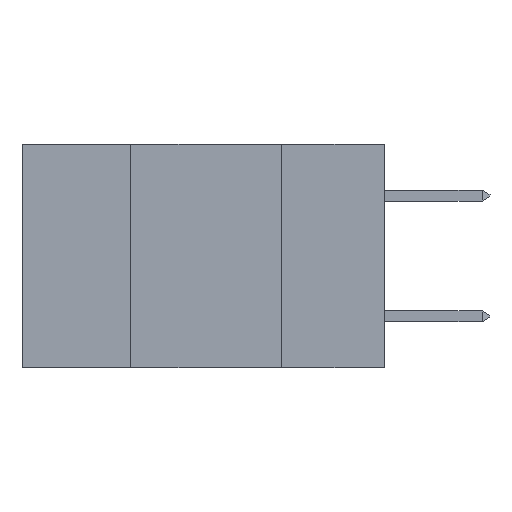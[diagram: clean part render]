
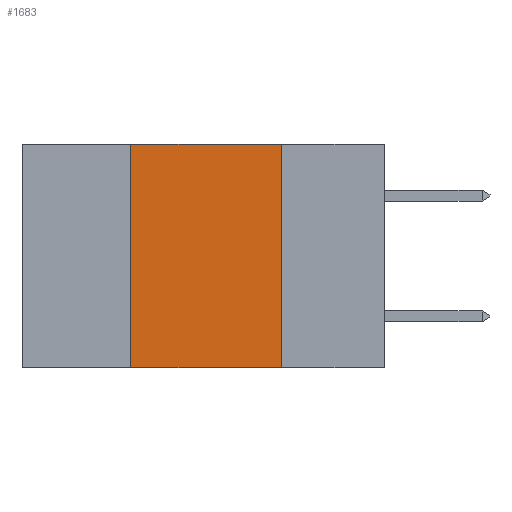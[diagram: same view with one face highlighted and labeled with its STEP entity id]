
A CAD part, left-side view. The second image highlights one B-rep face of the part: STEP entity #1683.
In plain terms, the highlighted planar face has unit normal (-1, 0, 0).
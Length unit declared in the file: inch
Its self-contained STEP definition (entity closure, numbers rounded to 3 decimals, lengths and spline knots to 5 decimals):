
#314 = CARTESIAN_POINT ( 'NONE',  ( 0., 0.42, 0. ) ) ;
#368 = VERTEX_POINT ( 'NONE', #5541 ) ;
#703 = CARTESIAN_POINT ( 'NONE',  ( 0., 0.17, 0. ) ) ;
#753 = CARTESIAN_POINT ( 'NONE',  ( 0., 0.6, -0.37 ) ) ;
#1014 = EDGE_CURVE ( 'NONE', #7011, #368, #11093, .T. ) ;
#1393 = VECTOR ( 'NONE', #2669, 39.37008 ) ;
#1591 = VERTEX_POINT ( 'NONE', #10261 ) ;
#1683 = ADVANCED_FACE ( 'NONE', ( #8081 ), #6097, .F. ) ;
#1705 = DIRECTION ( 'NONE',  ( 0., 0., -1. ) ) ;
#1725 = LINE ( 'NONE', #703, #8526 ) ;
#1885 = AXIS2_PLACEMENT_3D ( 'NONE', #4350, #7939, #2649 ) ;
#2500 = EDGE_CURVE ( 'NONE', #7571, #1591, #1725, .T. ) ;
#2526 = EDGE_CURVE ( 'NONE', #7011, #1591, #6122, .T. ) ;
#2649 = DIRECTION ( 'NONE',  ( 0., 0., -1. ) ) ;
#2669 = DIRECTION ( 'NONE',  ( 0., -1., 0. ) ) ;
#2849 = ORIENTED_EDGE ( 'NONE', *, *, #2500, .F. ) ;
#3360 = EDGE_CURVE ( 'NONE', #368, #7571, #3662, .T. ) ;
#3461 = CARTESIAN_POINT ( 'NONE',  ( 0., 0.42, -0.37 ) ) ;
#3528 = CARTESIAN_POINT ( 'NONE',  ( 0., 0.6, 0. ) ) ;
#3662 = LINE ( 'NONE', #3528, #10383 ) ;
#4350 = CARTESIAN_POINT ( 'NONE',  ( 0., 0.6, 0. ) ) ;
#5541 = CARTESIAN_POINT ( 'NONE',  ( 0., 0.42, 0. ) ) ;
#6097 = PLANE ( 'NONE',  #1885 ) ;
#6122 = LINE ( 'NONE', #753, #1393 ) ;
#6260 = ORIENTED_EDGE ( 'NONE', *, *, #3360, .F. ) ;
#6523 = ORIENTED_EDGE ( 'NONE', *, *, #2526, .T. ) ;
#6628 = DIRECTION ( 'NONE',  ( 0., 0., 1. ) ) ;
#7011 = VERTEX_POINT ( 'NONE', #3461 ) ;
#7454 = EDGE_LOOP ( 'NONE', ( #2849, #6260, #10955, #6523 ) ) ;
#7571 = VERTEX_POINT ( 'NONE', #9324 ) ;
#7939 = DIRECTION ( 'NONE',  ( 1., 0., 0. ) ) ;
#8081 = FACE_OUTER_BOUND ( 'NONE', #7454, .T. ) ;
#8526 = VECTOR ( 'NONE', #1705, 39.37008 ) ;
#8780 = VECTOR ( 'NONE', #6628, 39.37008 ) ;
#9324 = CARTESIAN_POINT ( 'NONE',  ( 0., 0.17, 0. ) ) ;
#10261 = CARTESIAN_POINT ( 'NONE',  ( 0., 0.17, -0.37 ) ) ;
#10383 = VECTOR ( 'NONE', #10550, 39.37008 ) ;
#10550 = DIRECTION ( 'NONE',  ( 0., -1., 0. ) ) ;
#10955 = ORIENTED_EDGE ( 'NONE', *, *, #1014, .F. ) ;
#11093 = LINE ( 'NONE', #314, #8780 ) ;
